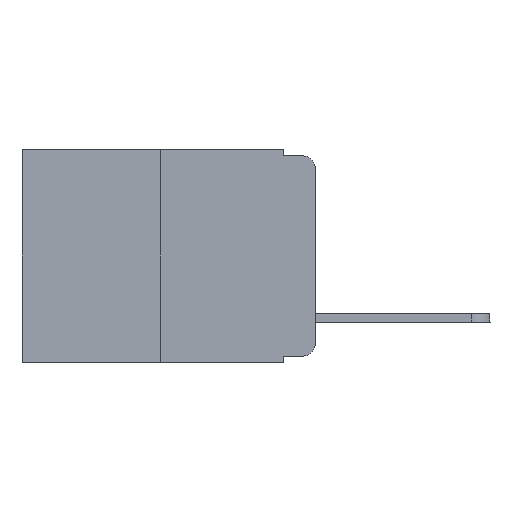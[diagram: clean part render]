
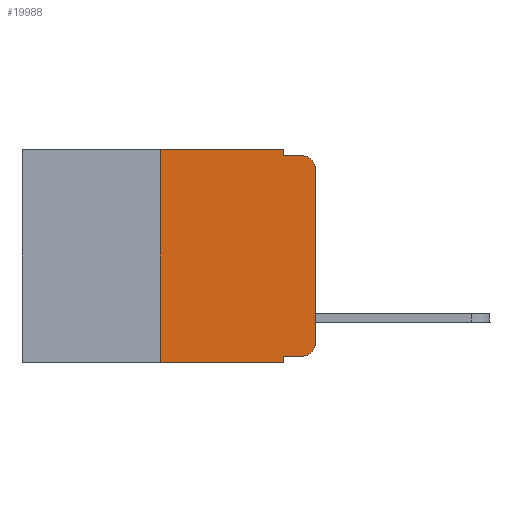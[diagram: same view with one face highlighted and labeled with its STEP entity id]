
A CAD part, left-side view. The second image highlights one B-rep face of the part: STEP entity #19988.
In plain terms, the highlighted planar face has unit normal (-1, 0, 0).
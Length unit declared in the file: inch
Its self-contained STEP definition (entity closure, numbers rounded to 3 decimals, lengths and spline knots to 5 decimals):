
#256 = CIRCLE ( 'NONE', #2903, 0.02 ) ;
#360 = CARTESIAN_POINT ( 'NONE',  ( 0., 0.02, -0.01 ) ) ;
#1385 = CARTESIAN_POINT ( 'NONE',  ( 0., 0.051, 0. ) ) ;
#2272 = VECTOR ( 'NONE', #10486, 39.37008 ) ;
#2467 = VERTEX_POINT ( 'NONE', #12586 ) ;
#2529 = DIRECTION ( 'NONE',  ( 0., 0., 1. ) ) ;
#2903 = AXIS2_PLACEMENT_3D ( 'NONE', #15038, #16608, #10293 ) ;
#3013 = ORIENTED_EDGE ( 'NONE', *, *, #6677, .F. ) ;
#3236 = CARTESIAN_POINT ( 'NONE',  ( 0., 0.02, -0.313 ) ) ;
#3307 = CARTESIAN_POINT ( 'NONE',  ( 0., 0.25, -0.343 ) ) ;
#3335 = LINE ( 'NONE', #12371, #4112 ) ;
#4112 = VECTOR ( 'NONE', #20236, 39.37008 ) ;
#4330 = AXIS2_PLACEMENT_3D ( 'NONE', #15872, #12498, #20720 ) ;
#4753 = VERTEX_POINT ( 'NONE', #6273 ) ;
#4765 = CARTESIAN_POINT ( 'NONE',  ( 0., 0., -0.313 ) ) ;
#4873 = DIRECTION ( 'NONE',  ( 0., 0., 1. ) ) ;
#4935 = DIRECTION ( 'NONE',  ( 0., -1., 0. ) ) ;
#5036 = VECTOR ( 'NONE', #2529, 39.37008 ) ;
#5233 = EDGE_CURVE ( 'NONE', #10005, #10982, #15220, .T. ) ;
#6178 = EDGE_CURVE ( 'NONE', #10005, #20243, #18523, .T. ) ;
#6273 = CARTESIAN_POINT ( 'NONE',  ( 0., 0., -0.03 ) ) ;
#6419 = EDGE_CURVE ( 'NONE', #10982, #13063, #18278, .T. ) ;
#6574 = CARTESIAN_POINT ( 'NONE',  ( 0., 0., 0. ) ) ;
#6677 = EDGE_CURVE ( 'NONE', #2467, #18365, #12915, .T. ) ;
#7819 = VECTOR ( 'NONE', #14853, 39.37008 ) ;
#8734 = CARTESIAN_POINT ( 'NONE',  ( 0., 0.25, 0. ) ) ;
#8911 = FACE_OUTER_BOUND ( 'NONE', #17628, .T. ) ;
#8973 = CARTESIAN_POINT ( 'NONE',  ( 0., 0.051, -0.333 ) ) ;
#9244 = DIRECTION ( 'NONE',  ( 0., 0., -1. ) ) ;
#9245 = CARTESIAN_POINT ( 'NONE',  ( 0., 0.051, -0.333 ) ) ;
#9416 = ORIENTED_EDGE ( 'NONE', *, *, #12224, .F. ) ;
#10005 = VERTEX_POINT ( 'NONE', #3307 ) ;
#10293 = DIRECTION ( 'NONE',  ( 0., 0., -1. ) ) ;
#10366 = LINE ( 'NONE', #8973, #11386 ) ;
#10486 = DIRECTION ( 'NONE',  ( 0., -1., 0. ) ) ;
#10496 = EDGE_CURVE ( 'NONE', #19531, #20243, #17887, .T. ) ;
#10616 = VERTEX_POINT ( 'NONE', #4765 ) ;
#10641 = CIRCLE ( 'NONE', #10794, 0.02 ) ;
#10794 = AXIS2_PLACEMENT_3D ( 'NONE', #3236, #11888, #9244 ) ;
#10866 = CARTESIAN_POINT ( 'NONE',  ( 0., 0.02, -0.333 ) ) ;
#10982 = VERTEX_POINT ( 'NONE', #15670 ) ;
#11102 = DIRECTION ( 'NONE',  ( 0., 0., -1. ) ) ;
#11386 = VECTOR ( 'NONE', #14927, 39.37008 ) ;
#11582 = ORIENTED_EDGE ( 'NONE', *, *, #6419, .F. ) ;
#11705 = ORIENTED_EDGE ( 'NONE', *, *, #15149, .T. ) ;
#11888 = DIRECTION ( 'NONE',  ( -1., 0., 0. ) ) ;
#12224 = EDGE_CURVE ( 'NONE', #13063, #2467, #3335, .T. ) ;
#12230 = LINE ( 'NONE', #6574, #20345 ) ;
#12371 = CARTESIAN_POINT ( 'NONE',  ( 0., 0.051, 0. ) ) ;
#12498 = DIRECTION ( 'NONE',  ( 1., 0., 0. ) ) ;
#12586 = CARTESIAN_POINT ( 'NONE',  ( 0., 0.051, -0.01 ) ) ;
#12849 = CARTESIAN_POINT ( 'NONE',  ( 0., 0.473, 0. ) ) ;
#12915 = LINE ( 'NONE', #18073, #7819 ) ;
#13063 = VERTEX_POINT ( 'NONE', #15691 ) ;
#13745 = VERTEX_POINT ( 'NONE', #10866 ) ;
#14145 = ORIENTED_EDGE ( 'NONE', *, *, #20126, .T. ) ;
#14819 = ORIENTED_EDGE ( 'NONE', *, *, #6178, .T. ) ;
#14853 = DIRECTION ( 'NONE',  ( 0., -1., 0. ) ) ;
#14927 = DIRECTION ( 'NONE',  ( 0., -1., 0. ) ) ;
#15038 = CARTESIAN_POINT ( 'NONE',  ( 0., 0.02, -0.03 ) ) ;
#15149 = EDGE_CURVE ( 'NONE', #4753, #18365, #256, .T. ) ;
#15220 = LINE ( 'NONE', #8734, #5036 ) ;
#15392 = EDGE_CURVE ( 'NONE', #13745, #10616, #10641, .T. ) ;
#15668 = CARTESIAN_POINT ( 'NONE',  ( 0., 0.473, -0.343 ) ) ;
#15670 = CARTESIAN_POINT ( 'NONE',  ( 0., 0.25, 0. ) ) ;
#15691 = CARTESIAN_POINT ( 'NONE',  ( 0., 0.051, 0. ) ) ;
#15872 = CARTESIAN_POINT ( 'NONE',  ( 0., 0.473, 0. ) ) ;
#16017 = EDGE_CURVE ( 'NONE', #19531, #13745, #10366, .T. ) ;
#16589 = CARTESIAN_POINT ( 'NONE',  ( 0., 0.051, -0.343 ) ) ;
#16608 = DIRECTION ( 'NONE',  ( -1., 0., 0. ) ) ;
#16848 = ORIENTED_EDGE ( 'NONE', *, *, #10496, .F. ) ;
#17594 = PLANE ( 'NONE',  #4330 ) ;
#17628 = EDGE_LOOP ( 'NONE', ( #14145, #11705, #3013, #9416, #11582, #17885, #14819, #16848, #20543, #19650 ) ) ;
#17647 = VECTOR ( 'NONE', #11102, 39.37008 ) ;
#17885 = ORIENTED_EDGE ( 'NONE', *, *, #5233, .F. ) ;
#17887 = LINE ( 'NONE', #1385, #17647 ) ;
#17995 = VECTOR ( 'NONE', #4935, 39.37008 ) ;
#18073 = CARTESIAN_POINT ( 'NONE',  ( 0., 0.051, -0.01 ) ) ;
#18278 = LINE ( 'NONE', #12849, #17995 ) ;
#18365 = VERTEX_POINT ( 'NONE', #360 ) ;
#18523 = LINE ( 'NONE', #15668, #2272 ) ;
#19531 = VERTEX_POINT ( 'NONE', #9245 ) ;
#19650 = ORIENTED_EDGE ( 'NONE', *, *, #15392, .T. ) ;
#19988 = ADVANCED_FACE ( 'NONE', ( #8911 ), #17594, .F. ) ;
#20126 = EDGE_CURVE ( 'NONE', #10616, #4753, #12230, .T. ) ;
#20236 = DIRECTION ( 'NONE',  ( 0., 0., -1. ) ) ;
#20243 = VERTEX_POINT ( 'NONE', #16589 ) ;
#20345 = VECTOR ( 'NONE', #4873, 39.37008 ) ;
#20543 = ORIENTED_EDGE ( 'NONE', *, *, #16017, .T. ) ;
#20720 = DIRECTION ( 'NONE',  ( 0., 0., -1. ) ) ;
